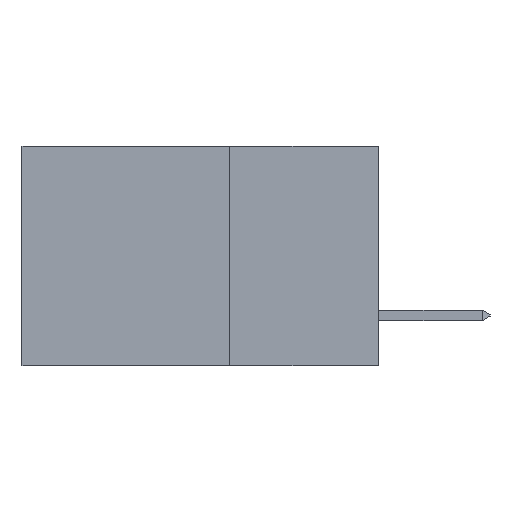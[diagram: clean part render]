
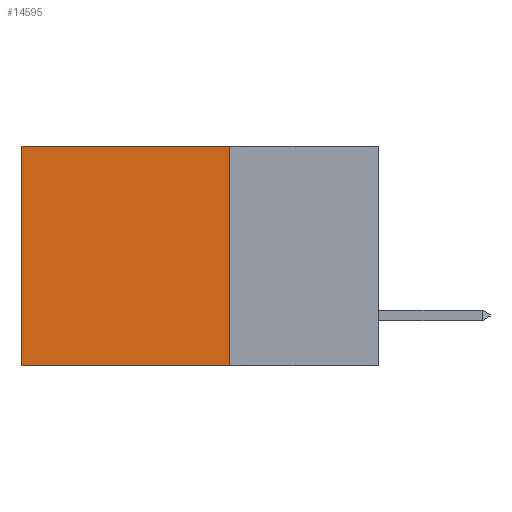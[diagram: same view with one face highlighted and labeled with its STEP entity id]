
A CAD part, left-side view. The second image highlights one B-rep face of the part: STEP entity #14595.
In plain terms, the highlighted planar face has unit normal (-1, 0, 0).
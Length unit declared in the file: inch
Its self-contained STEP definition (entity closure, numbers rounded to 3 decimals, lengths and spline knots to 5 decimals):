
#288 = ORIENTED_EDGE ( 'NONE', *, *, #18899, .F. ) ;
#2390 = VERTEX_POINT ( 'NONE', #7887 ) ;
#2427 = LINE ( 'NONE', #15689, #3031 ) ;
#3031 = VECTOR ( 'NONE', #4252, 39.37008 ) ;
#3850 = LINE ( 'NONE', #18792, #23387 ) ;
#4252 = DIRECTION ( 'NONE',  ( 0., 0., -1. ) ) ;
#4389 = LINE ( 'NONE', #8607, #23867 ) ;
#4461 = CARTESIAN_POINT ( 'NONE',  ( 0.298, 0.25, 0. ) ) ;
#4843 = DIRECTION ( 'NONE',  ( 0., 0., -1. ) ) ;
#5062 = FACE_OUTER_BOUND ( 'NONE', #19236, .T. ) ;
#5484 = DIRECTION ( 'NONE',  ( 0., 1., 0. ) ) ;
#7158 = EDGE_CURVE ( 'NONE', #2390, #20064, #9921, .T. ) ;
#7235 = DIRECTION ( 'NONE',  ( 1., 0., 0. ) ) ;
#7887 = CARTESIAN_POINT ( 'NONE',  ( 0.298, 0.25, 0. ) ) ;
#8263 = ORIENTED_EDGE ( 'NONE', *, *, #23491, .T. ) ;
#8509 = VERTEX_POINT ( 'NONE', #12643 ) ;
#8607 = CARTESIAN_POINT ( 'NONE',  ( 0.298, 0.25, -0.37 ) ) ;
#9921 = LINE ( 'NONE', #4461, #20019 ) ;
#10733 = CARTESIAN_POINT ( 'NONE',  ( 0.298, 0.6, -0.37 ) ) ;
#11662 = VERTEX_POINT ( 'NONE', #10733 ) ;
#12643 = CARTESIAN_POINT ( 'NONE',  ( 0.298, 0.6, 0. ) ) ;
#14395 = DIRECTION ( 'NONE',  ( 0., 1., 0. ) ) ;
#14525 = AXIS2_PLACEMENT_3D ( 'NONE', #18610, #7235, #20505 ) ;
#14595 = ADVANCED_FACE ( 'NONE', ( #5062 ), #22278, .F. ) ;
#15689 = CARTESIAN_POINT ( 'NONE',  ( 0.298, 0.6, 0. ) ) ;
#17022 = CARTESIAN_POINT ( 'NONE',  ( 0.298, 0.25, -0.37 ) ) ;
#17281 = EDGE_CURVE ( 'NONE', #2390, #8509, #3850, .T. ) ;
#18610 = CARTESIAN_POINT ( 'NONE',  ( 0.298, 0.25, 0. ) ) ;
#18792 = CARTESIAN_POINT ( 'NONE',  ( 0.298, 0.25, 0. ) ) ;
#18899 = EDGE_CURVE ( 'NONE', #20064, #11662, #4389, .T. ) ;
#19236 = EDGE_LOOP ( 'NONE', ( #8263, #288, #19475, #22327 ) ) ;
#19475 = ORIENTED_EDGE ( 'NONE', *, *, #7158, .F. ) ;
#20019 = VECTOR ( 'NONE', #4843, 39.37008 ) ;
#20064 = VERTEX_POINT ( 'NONE', #17022 ) ;
#20505 = DIRECTION ( 'NONE',  ( 0., 0., -1. ) ) ;
#22278 = PLANE ( 'NONE',  #14525 ) ;
#22327 = ORIENTED_EDGE ( 'NONE', *, *, #17281, .T. ) ;
#23387 = VECTOR ( 'NONE', #5484, 39.37008 ) ;
#23491 = EDGE_CURVE ( 'NONE', #8509, #11662, #2427, .T. ) ;
#23867 = VECTOR ( 'NONE', #14395, 39.37008 ) ;
